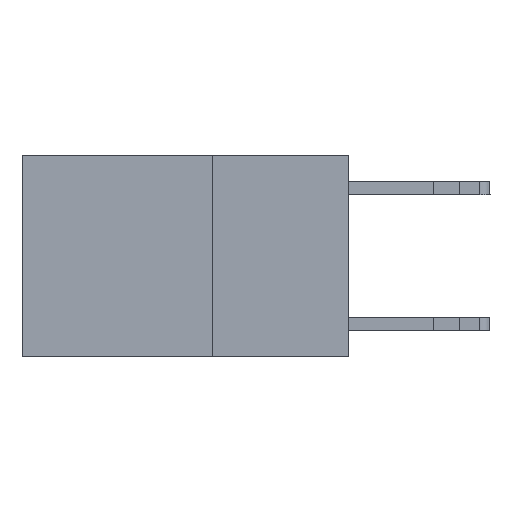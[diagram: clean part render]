
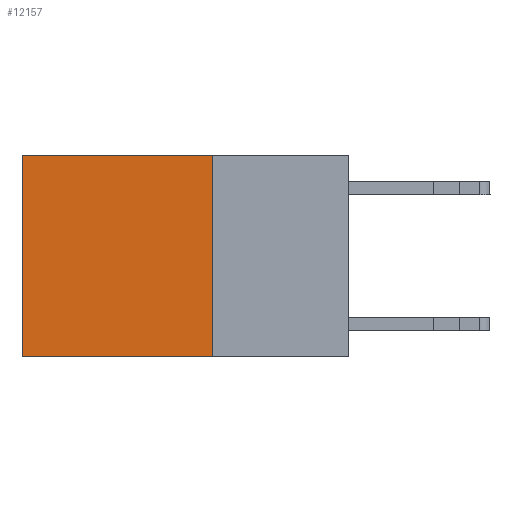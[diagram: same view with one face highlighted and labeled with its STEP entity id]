
A CAD part, left-side view. The second image highlights one B-rep face of the part: STEP entity #12157.
In plain terms, the highlighted planar face has unit normal (-1, 0, 0).
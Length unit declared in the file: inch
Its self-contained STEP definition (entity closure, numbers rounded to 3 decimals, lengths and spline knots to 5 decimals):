
#1471 = CARTESIAN_POINT ( 'NONE',  ( 0.2625, 0.25, 0. ) ) ;
#1668 = ORIENTED_EDGE ( 'NONE', *, *, #14357, .F. ) ;
#1877 = PLANE ( 'NONE',  #16088 ) ;
#1904 = VECTOR ( 'NONE', #8101, 39.37008 ) ;
#2567 = LINE ( 'NONE', #5923, #9430 ) ;
#5549 = LINE ( 'NONE', #17629, #1904 ) ;
#5576 = ORIENTED_EDGE ( 'NONE', *, *, #6221, .T. ) ;
#5628 = CARTESIAN_POINT ( 'NONE',  ( 0.2625, 0.25, 0. ) ) ;
#5923 = CARTESIAN_POINT ( 'NONE',  ( 0.2625, 0.25, 0. ) ) ;
#6202 = VECTOR ( 'NONE', #12419, 39.37008 ) ;
#6221 = EDGE_CURVE ( 'NONE', #9928, #11510, #5549, .T. ) ;
#6647 = EDGE_LOOP ( 'NONE', ( #5576, #1668, #12739, #17350 ) ) ;
#6708 = CARTESIAN_POINT ( 'NONE',  ( 0.2625, 0.25, -0.37 ) ) ;
#7189 = CARTESIAN_POINT ( 'NONE',  ( 0.2625, 0.6, 0. ) ) ;
#7312 = DIRECTION ( 'NONE',  ( 0., 0., -1. ) ) ;
#7390 = CARTESIAN_POINT ( 'NONE',  ( 0.2625, 0.25, 0. ) ) ;
#8063 = DIRECTION ( 'NONE',  ( 0., 1., 0. ) ) ;
#8101 = DIRECTION ( 'NONE',  ( 0., 0., -1. ) ) ;
#8618 = CARTESIAN_POINT ( 'NONE',  ( 0.2625, 0.25, -0.37 ) ) ;
#8775 = DIRECTION ( 'NONE',  ( 0., 0., -1. ) ) ;
#8850 = CARTESIAN_POINT ( 'NONE',  ( 0.2625, 0.6, -0.37 ) ) ;
#9430 = VECTOR ( 'NONE', #7312, 39.37008 ) ;
#9844 = LINE ( 'NONE', #1471, #6202 ) ;
#9928 = VERTEX_POINT ( 'NONE', #7189 ) ;
#10467 = LINE ( 'NONE', #6708, #17263 ) ;
#11403 = VERTEX_POINT ( 'NONE', #8618 ) ;
#11414 = EDGE_CURVE ( 'NONE', #13860, #11403, #2567, .T. ) ;
#11510 = VERTEX_POINT ( 'NONE', #8850 ) ;
#11873 = EDGE_CURVE ( 'NONE', #13860, #9928, #9844, .T. ) ;
#12157 = ADVANCED_FACE ( 'NONE', ( #12815 ), #1877, .F. ) ;
#12419 = DIRECTION ( 'NONE',  ( 0., 1., 0. ) ) ;
#12739 = ORIENTED_EDGE ( 'NONE', *, *, #11414, .F. ) ;
#12815 = FACE_OUTER_BOUND ( 'NONE', #6647, .T. ) ;
#13860 = VERTEX_POINT ( 'NONE', #5628 ) ;
#14357 = EDGE_CURVE ( 'NONE', #11403, #11510, #10467, .T. ) ;
#16088 = AXIS2_PLACEMENT_3D ( 'NONE', #7390, #16922, #8775 ) ;
#16922 = DIRECTION ( 'NONE',  ( 1., 0., 0. ) ) ;
#17263 = VECTOR ( 'NONE', #8063, 39.37008 ) ;
#17350 = ORIENTED_EDGE ( 'NONE', *, *, #11873, .T. ) ;
#17629 = CARTESIAN_POINT ( 'NONE',  ( 0.2625, 0.6, 0. ) ) ;
